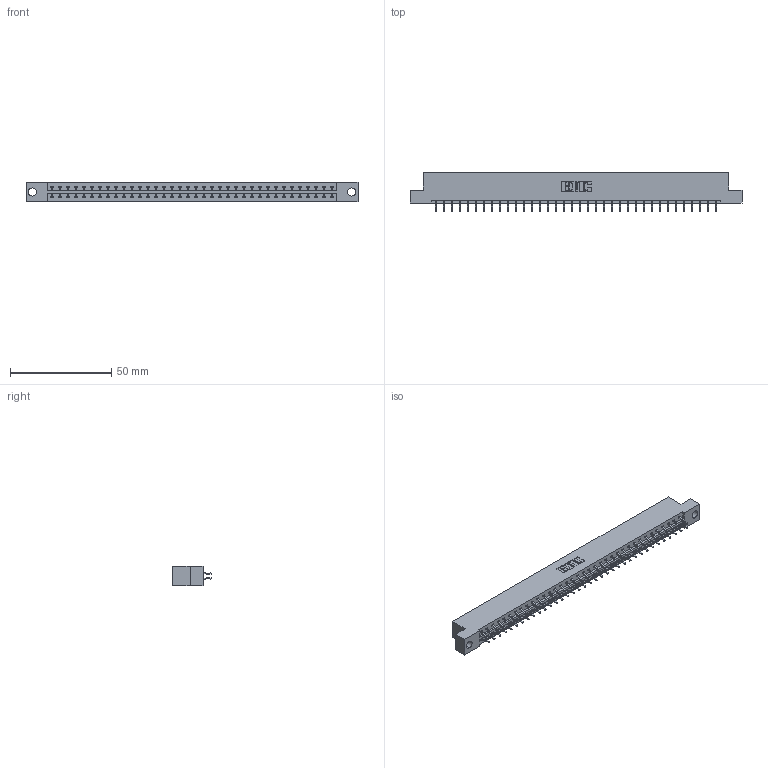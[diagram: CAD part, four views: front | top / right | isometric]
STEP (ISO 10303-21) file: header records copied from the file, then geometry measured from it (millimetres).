
FILE_DESCRIPTION (( 'STEP AP203' ), '1' );
FILE_NAME ('833-072-556-204.STEP', '2020-06-05T14:51:04', ( '' ), ( '' ), 'SwSTEP 2.0', 'SolidWorks 2020', '' );
FILE_SCHEMA (( 'CONFIG_CONTROL_DESIGN' ));
Length unit declared in the file: inch
Products named in the file (3): 345-292-001_556 Tail; 833 Part_Flush - .156 Dia - TH; 833-072-556-204
Assembly tree (73 placements, depth 2):
  833-072-556-204
    833 Part_Flush - .156 Dia - TH
    345-292-001_556 Tail  x72
Bounding box: 164.19 x 19.57 x 9.4 mm (x, y, z)
Volume: 16615.6 mm3; surface area: 19307.7 mm2
Topology: 73 solids, 73 shells, 4290 faces, 12767 edges, 8414 vertices
Faces by surface type: plane 2950, cylinder 1340
Entity records: 24159 total; most frequent: CARTESIAN_POINT 4026, ORIENTED_EDGE 3950, DIRECTION 3439, EDGE_CURVE 1975, LINE 1839, VECTOR 1839, VERTEX_POINT 1314, AXIS2_PLACEMENT_3D 800
